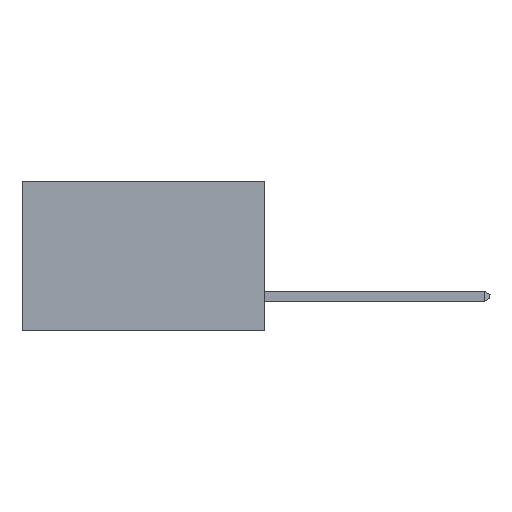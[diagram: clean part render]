
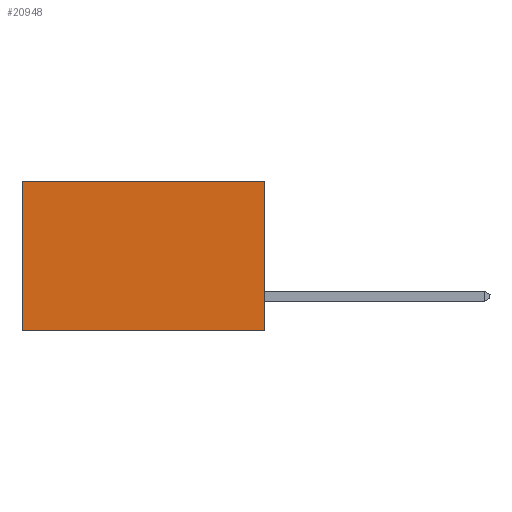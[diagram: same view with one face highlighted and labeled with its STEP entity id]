
A CAD part, left-side view. The second image highlights one B-rep face of the part: STEP entity #20948.
In plain terms, the highlighted planar face has unit normal (-1, 0, 0).
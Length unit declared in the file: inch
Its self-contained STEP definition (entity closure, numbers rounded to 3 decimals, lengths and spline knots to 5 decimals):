
#810 = AXIS2_PLACEMENT_3D ( 'NONE', #17279, #17215, #4005 ) ;
#1576 = CARTESIAN_POINT ( 'NONE',  ( 0.298, 0., 0. ) ) ;
#1920 = CARTESIAN_POINT ( 'NONE',  ( 0.298, 0., -0.37 ) ) ;
#2173 = DIRECTION ( 'NONE',  ( 0., 0., -1. ) ) ;
#2784 = CARTESIAN_POINT ( 'NONE',  ( 0.298, 0.6, 0. ) ) ;
#4005 = DIRECTION ( 'NONE',  ( 0., 0., -1. ) ) ;
#4204 = FACE_OUTER_BOUND ( 'NONE', #9473, .T. ) ;
#4403 = EDGE_CURVE ( 'NONE', #17511, #18290, #13246, .T. ) ;
#4669 = VECTOR ( 'NONE', #2173, 39.37008 ) ;
#5541 = PLANE ( 'NONE',  #810 ) ;
#7714 = ORIENTED_EDGE ( 'NONE', *, *, #4403, .F. ) ;
#7821 = CARTESIAN_POINT ( 'NONE',  ( 0.298, 0., -0.37 ) ) ;
#7967 = ORIENTED_EDGE ( 'NONE', *, *, #20496, .T. ) ;
#8085 = ORIENTED_EDGE ( 'NONE', *, *, #21636, .F. ) ;
#9258 = VERTEX_POINT ( 'NONE', #10494 ) ;
#9473 = EDGE_LOOP ( 'NONE', ( #13926, #8085, #7714, #7967 ) ) ;
#10494 = CARTESIAN_POINT ( 'NONE',  ( 0.298, 0.6, -0.37 ) ) ;
#10942 = CARTESIAN_POINT ( 'NONE',  ( 0.298, 0., 0. ) ) ;
#11059 = CARTESIAN_POINT ( 'NONE',  ( 0.298, 0., 0. ) ) ;
#11372 = VECTOR ( 'NONE', #12632, 39.37008 ) ;
#11518 = LINE ( 'NONE', #19090, #4669 ) ;
#11744 = DIRECTION ( 'NONE',  ( 0., 0., -1. ) ) ;
#12632 = DIRECTION ( 'NONE',  ( 0., 1., 0. ) ) ;
#13246 = LINE ( 'NONE', #1576, #13481 ) ;
#13481 = VECTOR ( 'NONE', #11744, 39.37008 ) ;
#13487 = DIRECTION ( 'NONE',  ( 0., 1., 0. ) ) ;
#13926 = ORIENTED_EDGE ( 'NONE', *, *, #20342, .T. ) ;
#14923 = VERTEX_POINT ( 'NONE', #2784 ) ;
#14929 = LINE ( 'NONE', #10942, #11372 ) ;
#16510 = LINE ( 'NONE', #1920, #17307 ) ;
#17215 = DIRECTION ( 'NONE',  ( 1., 0., 0. ) ) ;
#17279 = CARTESIAN_POINT ( 'NONE',  ( 0.298, 0., 0. ) ) ;
#17307 = VECTOR ( 'NONE', #13487, 39.37008 ) ;
#17511 = VERTEX_POINT ( 'NONE', #11059 ) ;
#18290 = VERTEX_POINT ( 'NONE', #7821 ) ;
#19090 = CARTESIAN_POINT ( 'NONE',  ( 0.298, 0.6, 0. ) ) ;
#20342 = EDGE_CURVE ( 'NONE', #14923, #9258, #11518, .T. ) ;
#20496 = EDGE_CURVE ( 'NONE', #17511, #14923, #14929, .T. ) ;
#20948 = ADVANCED_FACE ( 'NONE', ( #4204 ), #5541, .F. ) ;
#21636 = EDGE_CURVE ( 'NONE', #18290, #9258, #16510, .T. ) ;
